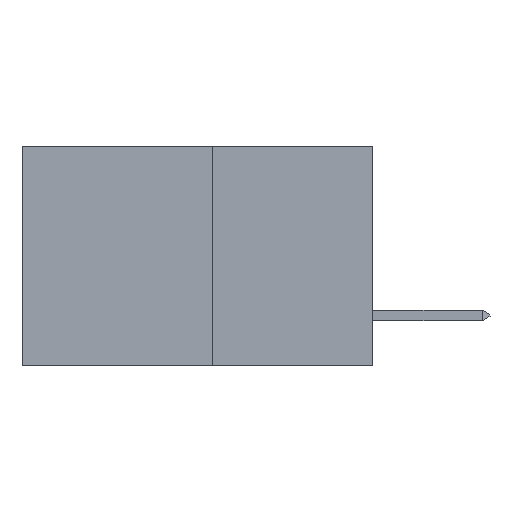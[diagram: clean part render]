
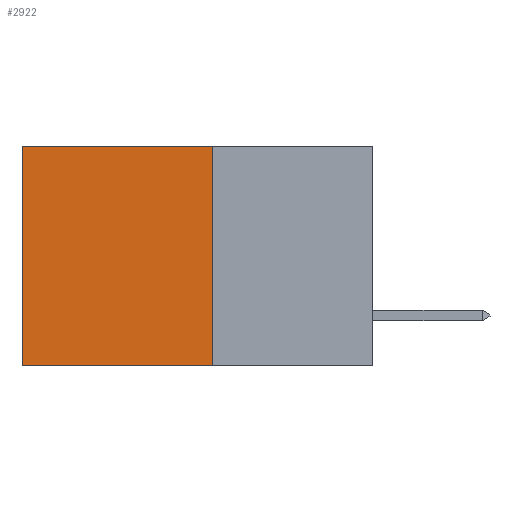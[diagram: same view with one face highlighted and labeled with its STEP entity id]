
A CAD part, left-side view. The second image highlights one B-rep face of the part: STEP entity #2922.
In plain terms, the highlighted planar face has unit normal (-1, 0, 0).
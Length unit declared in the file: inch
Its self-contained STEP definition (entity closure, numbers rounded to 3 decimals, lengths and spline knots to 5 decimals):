
#9 = VERTEX_POINT ( 'NONE', #8380 ) ;
#303 = DIRECTION ( 'NONE',  ( 0., 1., 0. ) ) ;
#399 = CARTESIAN_POINT ( 'NONE',  ( 0.277, 0.27, -0.37 ) ) ;
#1324 = CARTESIAN_POINT ( 'NONE',  ( 0.277, 0.27, -0.37 ) ) ;
#2161 = LINE ( 'NONE', #3636, #10674 ) ;
#2338 = EDGE_LOOP ( 'NONE', ( #4989, #5321, #5482, #5509 ) ) ;
#2922 = ADVANCED_FACE ( 'NONE', ( #4590 ), #9755, .F. ) ;
#3007 = VECTOR ( 'NONE', #303, 39.37008 ) ;
#3199 = AXIS2_PLACEMENT_3D ( 'NONE', #1324, #9642, #6575 ) ;
#3277 = VERTEX_POINT ( 'NONE', #7589 ) ;
#3556 = CARTESIAN_POINT ( 'NONE',  ( 0.277, 0.27, -0.37 ) ) ;
#3636 = CARTESIAN_POINT ( 'NONE',  ( 0.277, 0.59, -0.37 ) ) ;
#4116 = DIRECTION ( 'NONE',  ( 0., 0., -1. ) ) ;
#4137 = CARTESIAN_POINT ( 'NONE',  ( 0.277, 0.27, 0. ) ) ;
#4386 = VECTOR ( 'NONE', #9992, 39.37008 ) ;
#4590 = FACE_OUTER_BOUND ( 'NONE', #2338, .T. ) ;
#4878 = DIRECTION ( 'NONE',  ( 0., 1., 0. ) ) ;
#4989 = ORIENTED_EDGE ( 'NONE', *, *, #5667, .T. ) ;
#5321 = ORIENTED_EDGE ( 'NONE', *, *, #8662, .F. ) ;
#5441 = VERTEX_POINT ( 'NONE', #6261 ) ;
#5482 = ORIENTED_EDGE ( 'NONE', *, *, #7285, .F. ) ;
#5492 = EDGE_CURVE ( 'NONE', #5441, #9, #10548, .T. ) ;
#5509 = ORIENTED_EDGE ( 'NONE', *, *, #5492, .T. ) ;
#5667 = EDGE_CURVE ( 'NONE', #9, #3277, #2161, .T. ) ;
#6261 = CARTESIAN_POINT ( 'NONE',  ( 0.277, 0.27, 0. ) ) ;
#6575 = DIRECTION ( 'NONE',  ( 0., 0., -1. ) ) ;
#7285 = EDGE_CURVE ( 'NONE', #5441, #7570, #10634, .T. ) ;
#7570 = VERTEX_POINT ( 'NONE', #3556 ) ;
#7589 = CARTESIAN_POINT ( 'NONE',  ( 0.277, 0.59, -0.37 ) ) ;
#7762 = LINE ( 'NONE', #399, #3007 ) ;
#8212 = VECTOR ( 'NONE', #4878, 39.37008 ) ;
#8380 = CARTESIAN_POINT ( 'NONE',  ( 0.277, 0.59, 0. ) ) ;
#8662 = EDGE_CURVE ( 'NONE', #7570, #3277, #7762, .T. ) ;
#9642 = DIRECTION ( 'NONE',  ( 1., 0., 0. ) ) ;
#9755 = PLANE ( 'NONE',  #3199 ) ;
#9992 = DIRECTION ( 'NONE',  ( 0., 0., -1. ) ) ;
#10282 = CARTESIAN_POINT ( 'NONE',  ( 0.277, 0.27, -0.37 ) ) ;
#10548 = LINE ( 'NONE', #4137, #8212 ) ;
#10634 = LINE ( 'NONE', #10282, #4386 ) ;
#10674 = VECTOR ( 'NONE', #4116, 39.37008 ) ;
